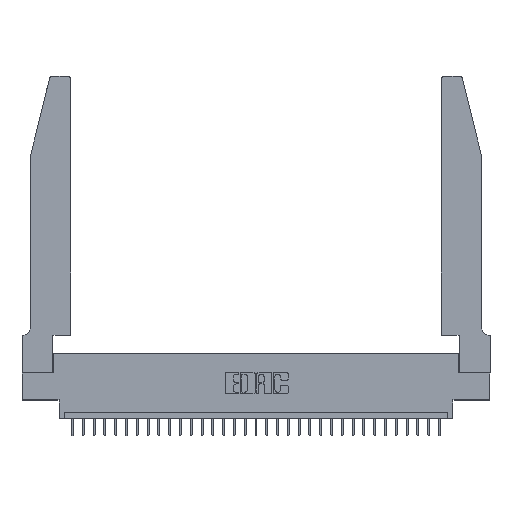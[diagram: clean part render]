
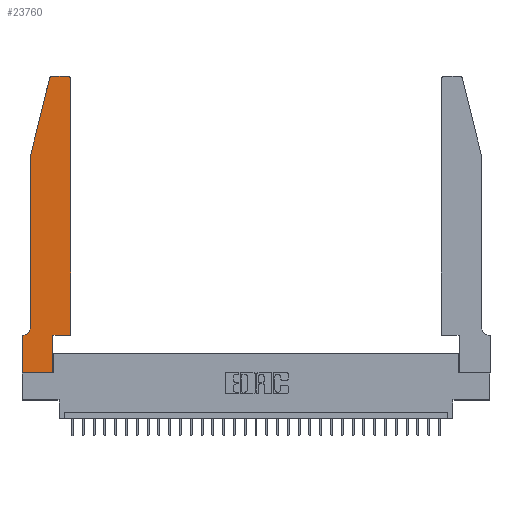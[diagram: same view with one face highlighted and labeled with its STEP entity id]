
A CAD part, top view. The second image highlights one B-rep face of the part: STEP entity #23760.
In plain terms, the highlighted planar face has unit normal (0, 0, 1).
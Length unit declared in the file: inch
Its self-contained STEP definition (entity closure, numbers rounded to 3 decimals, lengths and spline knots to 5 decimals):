
#276 = VECTOR ( 'NONE', #20267, 39.37008 ) ;
#781 = EDGE_CURVE ( 'NONE', #19522, #3907, #18105, .T. ) ;
#891 = PLANE ( 'NONE',  #11448 ) ;
#1245 = EDGE_CURVE ( 'NONE', #5027, #11764, #11130, .T. ) ;
#1459 = LINE ( 'NONE', #24917, #13537 ) ;
#1979 = CARTESIAN_POINT ( 'NONE',  ( 0.2605, 2.75, 0.37 ) ) ;
#2287 = CARTESIAN_POINT ( 'NONE',  ( 0., 0.35, 0.37 ) ) ;
#2305 = EDGE_LOOP ( 'NONE', ( #13801, #18875, #14315, #27264, #31986, #14019, #29896, #12369, #18037, #25034, #25188, #29073 ) ) ;
#3315 = DIRECTION ( 'NONE',  ( 1., 0., 0. ) ) ;
#3362 = CARTESIAN_POINT ( 'NONE',  ( 0., 0.35, 0.37 ) ) ;
#3841 = FACE_OUTER_BOUND ( 'NONE', #2305, .T. ) ;
#3907 = VERTEX_POINT ( 'NONE', #26562 ) ;
#4007 = EDGE_CURVE ( 'NONE', #9844, #24016, #27803, .T. ) ;
#4251 = EDGE_CURVE ( 'NONE', #15641, #6095, #21967, .T. ) ;
#4325 = EDGE_CURVE ( 'NONE', #17510, #19522, #22327, .T. ) ;
#4668 = VECTOR ( 'NONE', #7294, 39.37008 ) ;
#5027 = VERTEX_POINT ( 'NONE', #16653 ) ;
#5904 = CARTESIAN_POINT ( 'NONE',  ( 0., 0., 0.37 ) ) ;
#6058 = VECTOR ( 'NONE', #30800, 39.37008 ) ;
#6095 = VERTEX_POINT ( 'NONE', #8292 ) ;
#6564 = CARTESIAN_POINT ( 'NONE',  ( 0.0055, 0.42, 0.37 ) ) ;
#6999 = DIRECTION ( 'NONE',  ( -1., 0., 0. ) ) ;
#7294 = DIRECTION ( 'NONE',  ( -0.239, -0.971, 0. ) ) ;
#7865 = EDGE_CURVE ( 'NONE', #23350, #15641, #18567, .T. ) ;
#8292 = CARTESIAN_POINT ( 'NONE',  ( 0.4205, 2.75, 0.37 ) ) ;
#8420 = DIRECTION ( 'NONE',  ( 0., 0., 1. ) ) ;
#9378 = CARTESIAN_POINT ( 'NONE',  ( 0.2865, 0.35, 0.37 ) ) ;
#9412 = CARTESIAN_POINT ( 'NONE',  ( 0.0055, 0.35, 0.37 ) ) ;
#9644 = CARTESIAN_POINT ( 'NONE',  ( 0.2865, 0., 0.37 ) ) ;
#9844 = VERTEX_POINT ( 'NONE', #17057 ) ;
#9889 = VECTOR ( 'NONE', #19575, 39.37008 ) ;
#10292 = CIRCLE ( 'NONE', #16444, 0.07 ) ;
#10349 = EDGE_CURVE ( 'NONE', #6095, #5027, #18422, .T. ) ;
#11130 = CIRCLE ( 'NONE', #11617, 0.03 ) ;
#11448 = AXIS2_PLACEMENT_3D ( 'NONE', #3362, #23209, #18509 ) ;
#11617 = AXIS2_PLACEMENT_3D ( 'NONE', #21140, #31260, #28675 ) ;
#11764 = VERTEX_POINT ( 'NONE', #21938 ) ;
#11833 = VECTOR ( 'NONE', #6999, 39.37008 ) ;
#11973 = VECTOR ( 'NONE', #18970, 39.37008 ) ;
#12369 = ORIENTED_EDGE ( 'NONE', *, *, #4325, .T. ) ;
#12485 = CARTESIAN_POINT ( 'NONE',  ( 0.0755, 2., 0.37 ) ) ;
#13040 = CARTESIAN_POINT ( 'NONE',  ( 0.4505, 2.72, 0.37 ) ) ;
#13122 = CARTESIAN_POINT ( 'NONE',  ( 0., 0., 0.37 ) ) ;
#13327 = CARTESIAN_POINT ( 'NONE',  ( 0.4205, 2.72, 0.37 ) ) ;
#13537 = VECTOR ( 'NONE', #17054, 39.37008 ) ;
#13801 = ORIENTED_EDGE ( 'NONE', *, *, #10349, .T. ) ;
#14019 = ORIENTED_EDGE ( 'NONE', *, *, #31205, .T. ) ;
#14315 = ORIENTED_EDGE ( 'NONE', *, *, #29313, .T. ) ;
#14621 = CARTESIAN_POINT ( 'NONE',  ( 0.0755, 2., 0.37 ) ) ;
#14662 = EDGE_CURVE ( 'NONE', #22350, #17510, #30271, .T. ) ;
#15641 = VERTEX_POINT ( 'NONE', #13040 ) ;
#16444 = AXIS2_PLACEMENT_3D ( 'NONE', #6564, #28702, #26500 ) ;
#16653 = CARTESIAN_POINT ( 'NONE',  ( 0.284, 2.75, 0.37 ) ) ;
#16696 = VECTOR ( 'NONE', #25983, 39.37008 ) ;
#17054 = DIRECTION ( 'NONE',  ( 1., 0., 0. ) ) ;
#17057 = CARTESIAN_POINT ( 'NONE',  ( 0.0755, 2., 0.37 ) ) ;
#17510 = VERTEX_POINT ( 'NONE', #5904 ) ;
#17967 = CARTESIAN_POINT ( 'NONE',  ( 0.0755, 0.35, 0.37 ) ) ;
#18037 = ORIENTED_EDGE ( 'NONE', *, *, #781, .T. ) ;
#18060 = EDGE_CURVE ( 'NONE', #3907, #23350, #1459, .T. ) ;
#18105 = LINE ( 'NONE', #9378, #6058 ) ;
#18422 = LINE ( 'NONE', #1979, #11833 ) ;
#18509 = DIRECTION ( 'NONE',  ( 1., 0., 0. ) ) ;
#18567 = LINE ( 'NONE', #18866, #11973 ) ;
#18667 = CARTESIAN_POINT ( 'NONE',  ( 0.4505, 0.35, 0.37 ) ) ;
#18866 = CARTESIAN_POINT ( 'NONE',  ( 0.4505, 0.35, 0.37 ) ) ;
#18875 = ORIENTED_EDGE ( 'NONE', *, *, #1245, .T. ) ;
#18970 = DIRECTION ( 'NONE',  ( 0., 1., 0. ) ) ;
#19017 = LINE ( 'NONE', #17967, #276 ) ;
#19522 = VERTEX_POINT ( 'NONE', #9644 ) ;
#19575 = DIRECTION ( 'NONE',  ( 0., -1., 0. ) ) ;
#20078 = EDGE_CURVE ( 'NONE', #24016, #25843, #10292, .T. ) ;
#20242 = LINE ( 'NONE', #14621, #4668 ) ;
#20267 = DIRECTION ( 'NONE',  ( -1., 0., 0. ) ) ;
#20619 = CARTESIAN_POINT ( 'NONE',  ( 0., 0., 0.37 ) ) ;
#21140 = CARTESIAN_POINT ( 'NONE',  ( 0.284, 2.72, 0.37 ) ) ;
#21938 = CARTESIAN_POINT ( 'NONE',  ( 0.25487, 2.72718, 0.37 ) ) ;
#21967 = CIRCLE ( 'NONE', #24696, 0.03 ) ;
#22327 = LINE ( 'NONE', #13122, #30119 ) ;
#22350 = VERTEX_POINT ( 'NONE', #2287 ) ;
#23018 = DIRECTION ( 'NONE',  ( 1., 0., 0. ) ) ;
#23209 = DIRECTION ( 'NONE',  ( 0., 0., 1. ) ) ;
#23350 = VERTEX_POINT ( 'NONE', #18667 ) ;
#23760 = ADVANCED_FACE ( 'NONE', ( #3841 ), #891, .T. ) ;
#24016 = VERTEX_POINT ( 'NONE', #27179 ) ;
#24696 = AXIS2_PLACEMENT_3D ( 'NONE', #13327, #8420, #23018 ) ;
#24917 = CARTESIAN_POINT ( 'NONE',  ( 0.4505, 0.35, 0.37 ) ) ;
#25034 = ORIENTED_EDGE ( 'NONE', *, *, #18060, .T. ) ;
#25188 = ORIENTED_EDGE ( 'NONE', *, *, #7865, .T. ) ;
#25843 = VERTEX_POINT ( 'NONE', #9412 ) ;
#25983 = DIRECTION ( 'NONE',  ( 0., -1., 0. ) ) ;
#26500 = DIRECTION ( 'NONE',  ( -1., 0., 0. ) ) ;
#26562 = CARTESIAN_POINT ( 'NONE',  ( 0.2865, 0.35, 0.37 ) ) ;
#27179 = CARTESIAN_POINT ( 'NONE',  ( 0.0755, 0.42, 0.37 ) ) ;
#27264 = ORIENTED_EDGE ( 'NONE', *, *, #4007, .T. ) ;
#27803 = LINE ( 'NONE', #12485, #9889 ) ;
#28675 = DIRECTION ( 'NONE',  ( 1., 0., 0. ) ) ;
#28702 = DIRECTION ( 'NONE',  ( 0., 0., -1. ) ) ;
#29073 = ORIENTED_EDGE ( 'NONE', *, *, #4251, .T. ) ;
#29313 = EDGE_CURVE ( 'NONE', #11764, #9844, #20242, .T. ) ;
#29896 = ORIENTED_EDGE ( 'NONE', *, *, #14662, .T. ) ;
#30119 = VECTOR ( 'NONE', #3315, 39.37008 ) ;
#30271 = LINE ( 'NONE', #20619, #16696 ) ;
#30800 = DIRECTION ( 'NONE',  ( 0., 1., 0. ) ) ;
#31205 = EDGE_CURVE ( 'NONE', #25843, #22350, #19017, .T. ) ;
#31260 = DIRECTION ( 'NONE',  ( 0., 0., 1. ) ) ;
#31986 = ORIENTED_EDGE ( 'NONE', *, *, #20078, .T. ) ;
